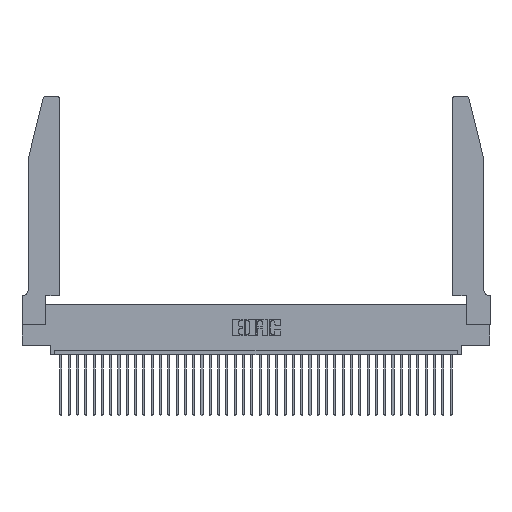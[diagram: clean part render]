
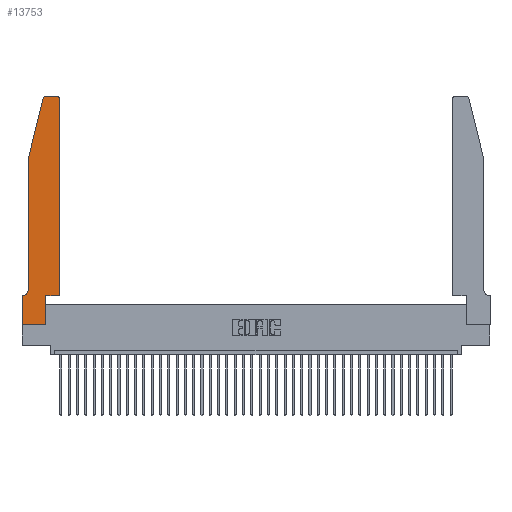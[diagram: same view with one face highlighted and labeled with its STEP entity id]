
A CAD part, top view. The second image highlights one B-rep face of the part: STEP entity #13753.
In plain terms, the highlighted planar face has unit normal (0, 0, 1).
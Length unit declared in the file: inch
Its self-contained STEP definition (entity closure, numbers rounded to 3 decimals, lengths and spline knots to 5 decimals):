
#135 = DIRECTION ( 'NONE',  ( 1., 0., 0. ) ) ;
#206 = LINE ( 'NONE', #19702, #5157 ) ;
#537 = AXIS2_PLACEMENT_3D ( 'NONE', #24099, #15397, #8888 ) ;
#822 = CARTESIAN_POINT ( 'NONE',  ( 0.4505, 0.35, 0.37 ) ) ;
#1150 = DIRECTION ( 'NONE',  ( -0.239, -0.971, 0. ) ) ;
#1637 = LINE ( 'NONE', #7517, #5531 ) ;
#2269 = ORIENTED_EDGE ( 'NONE', *, *, #34861, .T. ) ;
#2363 = LINE ( 'NONE', #14043, #2838 ) ;
#2466 = ORIENTED_EDGE ( 'NONE', *, *, #28777, .T. ) ;
#2560 = LINE ( 'NONE', #17191, #12730 ) ;
#2838 = VECTOR ( 'NONE', #20299, 39.37008 ) ;
#4174 = CARTESIAN_POINT ( 'NONE',  ( 0.2865, 0., 0.37 ) ) ;
#4197 = VECTOR ( 'NONE', #8633, 39.37008 ) ;
#4220 = CARTESIAN_POINT ( 'NONE',  ( 0.4505, 0.35, 0.37 ) ) ;
#4604 = CARTESIAN_POINT ( 'NONE',  ( 0.0755, 2., 0.37 ) ) ;
#5157 = VECTOR ( 'NONE', #13323, 39.37008 ) ;
#5531 = VECTOR ( 'NONE', #1150, 39.37008 ) ;
#6129 = EDGE_CURVE ( 'NONE', #26004, #29478, #2560, .T. ) ;
#6216 = CARTESIAN_POINT ( 'NONE',  ( 0.0055, 0.42, 0.37 ) ) ;
#7332 = AXIS2_PLACEMENT_3D ( 'NONE', #6216, #25612, #37333 ) ;
#7517 = CARTESIAN_POINT ( 'NONE',  ( 0.0755, 2., 0.37 ) ) ;
#7618 = VECTOR ( 'NONE', #39994, 39.37008 ) ;
#7660 = ORIENTED_EDGE ( 'NONE', *, *, #35864, .T. ) ;
#7803 = CARTESIAN_POINT ( 'NONE',  ( 0.2865, 0.35, 0.37 ) ) ;
#7839 = CARTESIAN_POINT ( 'NONE',  ( 0., 0., 0.37 ) ) ;
#8023 = PLANE ( 'NONE',  #14188 ) ;
#8161 = DIRECTION ( 'NONE',  ( 1., 0., 0. ) ) ;
#8267 = CIRCLE ( 'NONE', #7332, 0.07 ) ;
#8434 = EDGE_CURVE ( 'NONE', #39673, #19017, #2363, .T. ) ;
#8446 = VERTEX_POINT ( 'NONE', #11202 ) ;
#8633 = DIRECTION ( 'NONE',  ( -1., 0., 0. ) ) ;
#8888 = DIRECTION ( 'NONE',  ( 1., 0., 0. ) ) ;
#9912 = ORIENTED_EDGE ( 'NONE', *, *, #31824, .T. ) ;
#10317 = DIRECTION ( 'NONE',  ( 0., 1., 0. ) ) ;
#10516 = LINE ( 'NONE', #36454, #4197 ) ;
#11173 = LINE ( 'NONE', #28807, #11641 ) ;
#11202 = CARTESIAN_POINT ( 'NONE',  ( 0.0755, 0.42, 0.37 ) ) ;
#11641 = VECTOR ( 'NONE', #10317, 39.37008 ) ;
#11943 = VECTOR ( 'NONE', #16868, 39.37008 ) ;
#12054 = CARTESIAN_POINT ( 'NONE',  ( 0.4505, 2.72, 0.37 ) ) ;
#12248 = EDGE_CURVE ( 'NONE', #25680, #21115, #11173, .T. ) ;
#12428 = CARTESIAN_POINT ( 'NONE',  ( 0., 0., 0.37 ) ) ;
#12463 = VERTEX_POINT ( 'NONE', #35809 ) ;
#12730 = VECTOR ( 'NONE', #21358, 39.37008 ) ;
#13323 = DIRECTION ( 'NONE',  ( -1., 0., 0. ) ) ;
#13351 = EDGE_CURVE ( 'NONE', #38591, #39673, #10516, .T. ) ;
#13753 = ADVANCED_FACE ( 'NONE', ( #18316 ), #8023, .T. ) ;
#14043 = CARTESIAN_POINT ( 'NONE',  ( 0., 0., 0.37 ) ) ;
#14188 = AXIS2_PLACEMENT_3D ( 'NONE', #27024, #35999, #8161 ) ;
#14217 = EDGE_CURVE ( 'NONE', #19017, #25680, #22643, .T. ) ;
#14311 = CIRCLE ( 'NONE', #21905, 0.03 ) ;
#15331 = LINE ( 'NONE', #822, #11943 ) ;
#15397 = DIRECTION ( 'NONE',  ( 0., 0., 1. ) ) ;
#15648 = CARTESIAN_POINT ( 'NONE',  ( 0.284, 2.72, 0.37 ) ) ;
#15782 = ORIENTED_EDGE ( 'NONE', *, *, #12248, .T. ) ;
#15800 = CIRCLE ( 'NONE', #537, 0.03 ) ;
#16526 = LINE ( 'NONE', #4604, #39842 ) ;
#16868 = DIRECTION ( 'NONE',  ( 1., 0., 0. ) ) ;
#16996 = ORIENTED_EDGE ( 'NONE', *, *, #13351, .T. ) ;
#17191 = CARTESIAN_POINT ( 'NONE',  ( 0.4505, 0.35, 0.37 ) ) ;
#18316 = FACE_OUTER_BOUND ( 'NONE', #25835, .T. ) ;
#19017 = VERTEX_POINT ( 'NONE', #7839 ) ;
#19328 = ORIENTED_EDGE ( 'NONE', *, *, #34455, .T. ) ;
#19702 = CARTESIAN_POINT ( 'NONE',  ( 0.2605, 2.75, 0.37 ) ) ;
#20299 = DIRECTION ( 'NONE',  ( 0., -1., 0. ) ) ;
#20302 = VERTEX_POINT ( 'NONE', #33954 ) ;
#21065 = ORIENTED_EDGE ( 'NONE', *, *, #8434, .T. ) ;
#21115 = VERTEX_POINT ( 'NONE', #7803 ) ;
#21255 = ORIENTED_EDGE ( 'NONE', *, *, #14217, .T. ) ;
#21342 = EDGE_CURVE ( 'NONE', #8446, #38591, #8267, .T. ) ;
#21358 = DIRECTION ( 'NONE',  ( 0., 1., 0. ) ) ;
#21905 = AXIS2_PLACEMENT_3D ( 'NONE', #15648, #22386, #135 ) ;
#22386 = DIRECTION ( 'NONE',  ( 0., 0., 1. ) ) ;
#22612 = VERTEX_POINT ( 'NONE', #35965 ) ;
#22643 = LINE ( 'NONE', #12428, #7618 ) ;
#24099 = CARTESIAN_POINT ( 'NONE',  ( 0.4205, 2.72, 0.37 ) ) ;
#24363 = VERTEX_POINT ( 'NONE', #32412 ) ;
#24766 = ORIENTED_EDGE ( 'NONE', *, *, #21342, .T. ) ;
#25612 = DIRECTION ( 'NONE',  ( 0., 0., -1. ) ) ;
#25680 = VERTEX_POINT ( 'NONE', #4174 ) ;
#25835 = EDGE_LOOP ( 'NONE', ( #2466, #7660, #28524, #9912, #24766, #16996, #21065, #21255, #15782, #2269, #37760, #19328 ) ) ;
#26004 = VERTEX_POINT ( 'NONE', #4220 ) ;
#27024 = CARTESIAN_POINT ( 'NONE',  ( 0., 0.35, 0.37 ) ) ;
#28524 = ORIENTED_EDGE ( 'NONE', *, *, #29639, .T. ) ;
#28777 = EDGE_CURVE ( 'NONE', #20302, #24363, #206, .T. ) ;
#28807 = CARTESIAN_POINT ( 'NONE',  ( 0.2865, 0.35, 0.37 ) ) ;
#29478 = VERTEX_POINT ( 'NONE', #12054 ) ;
#29605 = DIRECTION ( 'NONE',  ( 0., -1., 0. ) ) ;
#29639 = EDGE_CURVE ( 'NONE', #12463, #22612, #1637, .T. ) ;
#31387 = CARTESIAN_POINT ( 'NONE',  ( 0., 0.35, 0.37 ) ) ;
#31824 = EDGE_CURVE ( 'NONE', #22612, #8446, #16526, .T. ) ;
#32412 = CARTESIAN_POINT ( 'NONE',  ( 0.284, 2.75, 0.37 ) ) ;
#33954 = CARTESIAN_POINT ( 'NONE',  ( 0.4205, 2.75, 0.37 ) ) ;
#34455 = EDGE_CURVE ( 'NONE', #29478, #20302, #15800, .T. ) ;
#34861 = EDGE_CURVE ( 'NONE', #21115, #26004, #15331, .T. ) ;
#35809 = CARTESIAN_POINT ( 'NONE',  ( 0.25487, 2.72718, 0.37 ) ) ;
#35864 = EDGE_CURVE ( 'NONE', #24363, #12463, #14311, .T. ) ;
#35965 = CARTESIAN_POINT ( 'NONE',  ( 0.0755, 2., 0.37 ) ) ;
#35999 = DIRECTION ( 'NONE',  ( 0., 0., 1. ) ) ;
#36454 = CARTESIAN_POINT ( 'NONE',  ( 0.0755, 0.35, 0.37 ) ) ;
#36653 = CARTESIAN_POINT ( 'NONE',  ( 0.0055, 0.35, 0.37 ) ) ;
#37333 = DIRECTION ( 'NONE',  ( -1., 0., 0. ) ) ;
#37760 = ORIENTED_EDGE ( 'NONE', *, *, #6129, .T. ) ;
#38591 = VERTEX_POINT ( 'NONE', #36653 ) ;
#39673 = VERTEX_POINT ( 'NONE', #31387 ) ;
#39842 = VECTOR ( 'NONE', #29605, 39.37008 ) ;
#39994 = DIRECTION ( 'NONE',  ( 1., 0., 0. ) ) ;
